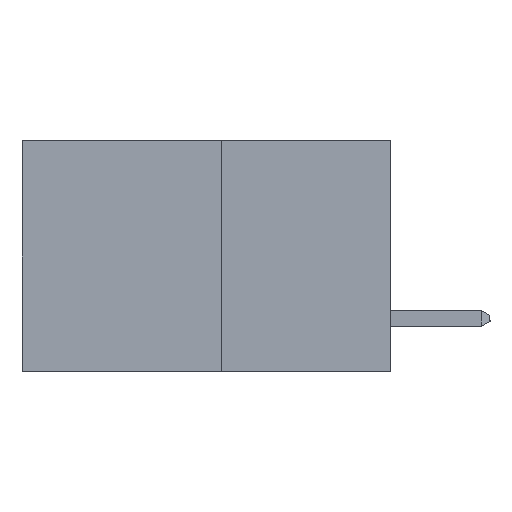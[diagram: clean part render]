
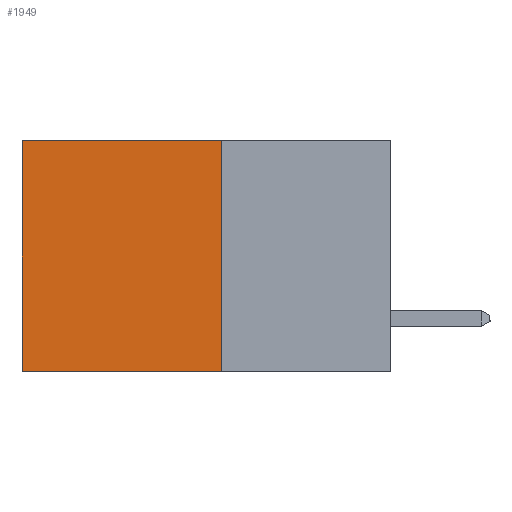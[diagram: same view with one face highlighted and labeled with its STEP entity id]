
A CAD part, left-side view. The second image highlights one B-rep face of the part: STEP entity #1949.
In plain terms, the highlighted planar face has unit normal (-1, 0, 0).
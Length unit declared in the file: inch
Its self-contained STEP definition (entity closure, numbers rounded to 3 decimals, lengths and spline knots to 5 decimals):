
#556 = VERTEX_POINT ( 'NONE', #5738 ) ;
#951 = FACE_OUTER_BOUND ( 'NONE', #14321, .T. ) ;
#1353 = VERTEX_POINT ( 'NONE', #13480 ) ;
#1949 = ADVANCED_FACE ( 'NONE', ( #951 ), #10431, .F. ) ;
#2193 = DIRECTION ( 'NONE',  ( 0., 0., -1. ) ) ;
#2194 = CARTESIAN_POINT ( 'NONE',  ( 0.277, 0.27, 0. ) ) ;
#2234 = CARTESIAN_POINT ( 'NONE',  ( 0.277, 0.59, -0.37 ) ) ;
#2740 = VECTOR ( 'NONE', #2193, 39.37008 ) ;
#4100 = EDGE_CURVE ( 'NONE', #556, #6467, #13305, .T. ) ;
#4667 = EDGE_CURVE ( 'NONE', #13734, #556, #5205, .T. ) ;
#4824 = ORIENTED_EDGE ( 'NONE', *, *, #4836, .T. ) ;
#4836 = EDGE_CURVE ( 'NONE', #1353, #6467, #5761, .T. ) ;
#4847 = VECTOR ( 'NONE', #5420, 39.37008 ) ;
#5205 = LINE ( 'NONE', #5872, #4847 ) ;
#5420 = DIRECTION ( 'NONE',  ( 0., 0., -1. ) ) ;
#5738 = CARTESIAN_POINT ( 'NONE',  ( 0.277, 0.27, -0.37 ) ) ;
#5761 = LINE ( 'NONE', #2234, #2740 ) ;
#5872 = CARTESIAN_POINT ( 'NONE',  ( 0.277, 0.27, -0.37 ) ) ;
#6202 = AXIS2_PLACEMENT_3D ( 'NONE', #10310, #10409, #10392 ) ;
#6467 = VERTEX_POINT ( 'NONE', #11238 ) ;
#6515 = VECTOR ( 'NONE', #7860, 39.37008 ) ;
#7191 = CARTESIAN_POINT ( 'NONE',  ( 0.277, 0.27, 0. ) ) ;
#7860 = DIRECTION ( 'NONE',  ( 0., 1., 0. ) ) ;
#8155 = ORIENTED_EDGE ( 'NONE', *, *, #4100, .F. ) ;
#8598 = DIRECTION ( 'NONE',  ( 0., 1., 0. ) ) ;
#9057 = CARTESIAN_POINT ( 'NONE',  ( 0.277, 0.27, -0.37 ) ) ;
#10310 = CARTESIAN_POINT ( 'NONE',  ( 0.277, 0.27, -0.37 ) ) ;
#10344 = VECTOR ( 'NONE', #8598, 39.37008 ) ;
#10392 = DIRECTION ( 'NONE',  ( 0., 0., -1. ) ) ;
#10409 = DIRECTION ( 'NONE',  ( 1., 0., 0. ) ) ;
#10431 = PLANE ( 'NONE',  #6202 ) ;
#10480 = ORIENTED_EDGE ( 'NONE', *, *, #12190, .T. ) ;
#11238 = CARTESIAN_POINT ( 'NONE',  ( 0.277, 0.59, -0.37 ) ) ;
#12190 = EDGE_CURVE ( 'NONE', #13734, #1353, #12461, .T. ) ;
#12461 = LINE ( 'NONE', #2194, #6515 ) ;
#13305 = LINE ( 'NONE', #9057, #10344 ) ;
#13480 = CARTESIAN_POINT ( 'NONE',  ( 0.277, 0.59, 0. ) ) ;
#13734 = VERTEX_POINT ( 'NONE', #7191 ) ;
#14118 = ORIENTED_EDGE ( 'NONE', *, *, #4667, .F. ) ;
#14321 = EDGE_LOOP ( 'NONE', ( #4824, #8155, #14118, #10480 ) ) ;
